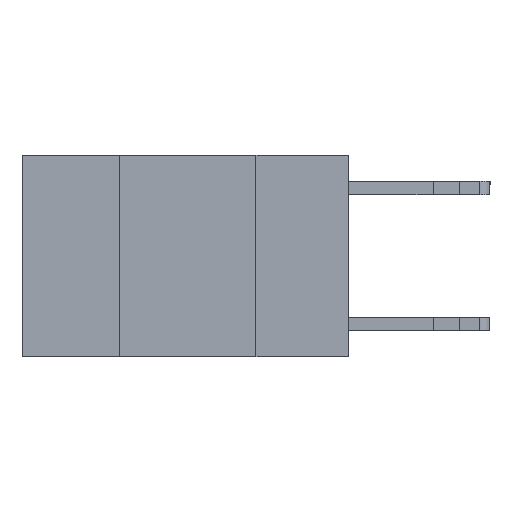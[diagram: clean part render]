
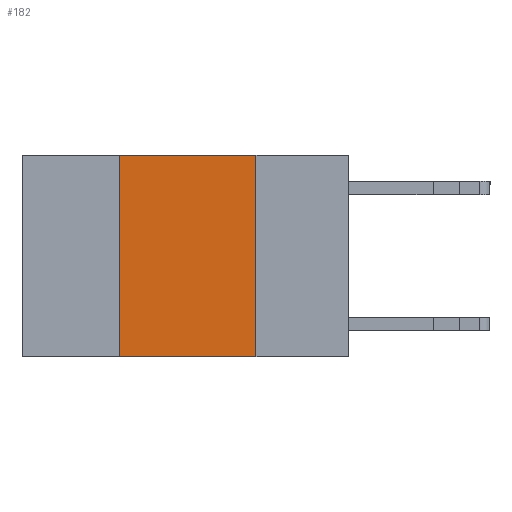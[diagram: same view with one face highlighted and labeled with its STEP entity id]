
A CAD part, left-side view. The second image highlights one B-rep face of the part: STEP entity #182.
In plain terms, the highlighted planar face has unit normal (-1, 0, 0).
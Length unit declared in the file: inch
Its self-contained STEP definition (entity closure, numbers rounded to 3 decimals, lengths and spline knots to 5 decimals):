
#182 = ADVANCED_FACE ( 'NONE', ( #13783 ), #11772, .F. ) ;
#427 = DIRECTION ( 'NONE',  ( 0., 0., -1. ) ) ;
#735 = LINE ( 'NONE', #16122, #4648 ) ;
#1070 = LINE ( 'NONE', #18101, #13759 ) ;
#3930 = ORIENTED_EDGE ( 'NONE', *, *, #12740, .F. ) ;
#4648 = VECTOR ( 'NONE', #23951, 39.37008 ) ;
#6085 = DIRECTION ( 'NONE',  ( 1., 0., 0. ) ) ;
#6086 = EDGE_CURVE ( 'NONE', #18956, #15094, #24543, .T. ) ;
#6183 = DIRECTION ( 'NONE',  ( 0., 0., 1. ) ) ;
#6254 = ORIENTED_EDGE ( 'NONE', *, *, #6086, .T. ) ;
#6556 = LINE ( 'NONE', #11993, #11112 ) ;
#7114 = VECTOR ( 'NONE', #10905, 39.37008 ) ;
#8784 = CARTESIAN_POINT ( 'NONE',  ( 0., 0.6, -0.37 ) ) ;
#9584 = CARTESIAN_POINT ( 'NONE',  ( 0., 0.17, 0. ) ) ;
#10673 = CARTESIAN_POINT ( 'NONE',  ( 0., 0.42, 0. ) ) ;
#10763 = DIRECTION ( 'NONE',  ( 0., -1., 0. ) ) ;
#10905 = DIRECTION ( 'NONE',  ( 0., -1., 0. ) ) ;
#11112 = VECTOR ( 'NONE', #6183, 39.37008 ) ;
#11772 = PLANE ( 'NONE',  #17023 ) ;
#11993 = CARTESIAN_POINT ( 'NONE',  ( 0., 0.42, 0. ) ) ;
#12649 = ORIENTED_EDGE ( 'NONE', *, *, #22750, .F. ) ;
#12740 = EDGE_CURVE ( 'NONE', #18956, #21572, #6556, .T. ) ;
#13041 = VERTEX_POINT ( 'NONE', #9584 ) ;
#13667 = CARTESIAN_POINT ( 'NONE',  ( 0., 0.6, 0. ) ) ;
#13759 = VECTOR ( 'NONE', #10763, 39.37008 ) ;
#13783 = FACE_OUTER_BOUND ( 'NONE', #18899, .T. ) ;
#14516 = CARTESIAN_POINT ( 'NONE',  ( 0., 0.42, -0.37 ) ) ;
#15094 = VERTEX_POINT ( 'NONE', #20024 ) ;
#16122 = CARTESIAN_POINT ( 'NONE',  ( 0., 0.17, 0. ) ) ;
#16188 = ORIENTED_EDGE ( 'NONE', *, *, #16601, .F. ) ;
#16601 = EDGE_CURVE ( 'NONE', #21572, #13041, #1070, .T. ) ;
#17023 = AXIS2_PLACEMENT_3D ( 'NONE', #13667, #6085, #427 ) ;
#18101 = CARTESIAN_POINT ( 'NONE',  ( 0., 0.6, 0. ) ) ;
#18899 = EDGE_LOOP ( 'NONE', ( #12649, #16188, #3930, #6254 ) ) ;
#18956 = VERTEX_POINT ( 'NONE', #14516 ) ;
#20024 = CARTESIAN_POINT ( 'NONE',  ( 0., 0.17, -0.37 ) ) ;
#21572 = VERTEX_POINT ( 'NONE', #10673 ) ;
#22750 = EDGE_CURVE ( 'NONE', #13041, #15094, #735, .T. ) ;
#23951 = DIRECTION ( 'NONE',  ( 0., 0., -1. ) ) ;
#24543 = LINE ( 'NONE', #8784, #7114 ) ;
